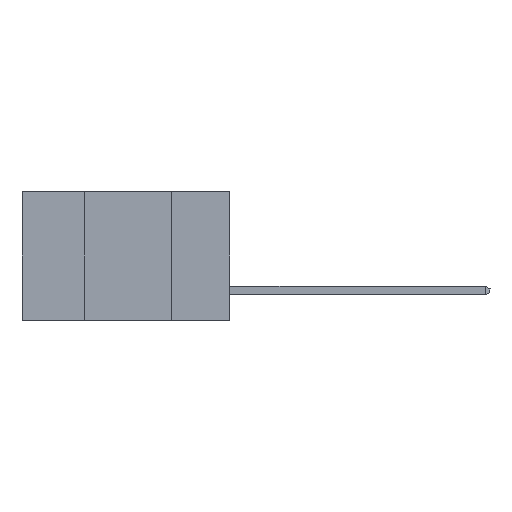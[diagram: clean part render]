
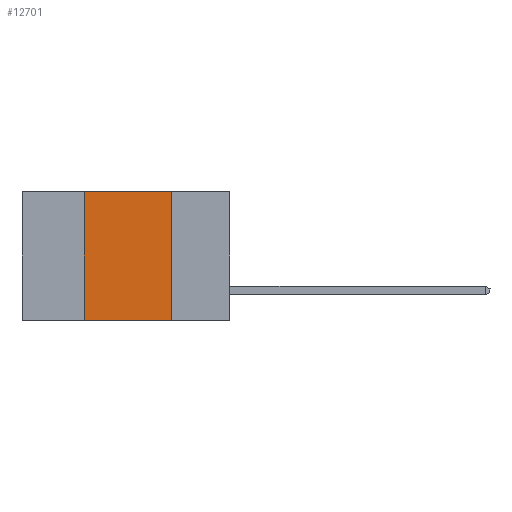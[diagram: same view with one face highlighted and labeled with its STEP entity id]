
A CAD part, left-side view. The second image highlights one B-rep face of the part: STEP entity #12701.
In plain terms, the highlighted planar face has unit normal (-1, 0, 0).
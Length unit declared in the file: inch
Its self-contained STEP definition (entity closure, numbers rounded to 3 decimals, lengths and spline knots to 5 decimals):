
#995 = DIRECTION ( 'NONE',  ( 0., 0., -1. ) ) ;
#1288 = CARTESIAN_POINT ( 'NONE',  ( 0., 0.42, 0. ) ) ;
#1943 = LINE ( 'NONE', #11636, #4097 ) ;
#1996 = DIRECTION ( 'NONE',  ( 0., 0., -1. ) ) ;
#2023 = CARTESIAN_POINT ( 'NONE',  ( 0., 0.42, -0.37 ) ) ;
#2169 = CARTESIAN_POINT ( 'NONE',  ( 0., 0.6, 0. ) ) ;
#2210 = LINE ( 'NONE', #11900, #9427 ) ;
#2412 = EDGE_CURVE ( 'NONE', #7372, #12033, #1943, .T. ) ;
#2417 = VECTOR ( 'NONE', #4695, 39.37008 ) ;
#2728 = ORIENTED_EDGE ( 'NONE', *, *, #10394, .F. ) ;
#3647 = EDGE_LOOP ( 'NONE', ( #7313, #10291, #2728, #4314 ) ) ;
#3679 = CARTESIAN_POINT ( 'NONE',  ( 0., 0.6, 0. ) ) ;
#3912 = CARTESIAN_POINT ( 'NONE',  ( 0., 0.17, -0.37 ) ) ;
#4097 = VECTOR ( 'NONE', #5203, 39.37008 ) ;
#4314 = ORIENTED_EDGE ( 'NONE', *, *, #2412, .T. ) ;
#4695 = DIRECTION ( 'NONE',  ( 0., -1., 0. ) ) ;
#5203 = DIRECTION ( 'NONE',  ( 0., -1., 0. ) ) ;
#6564 = LINE ( 'NONE', #7814, #9558 ) ;
#6735 = EDGE_CURVE ( 'NONE', #7533, #10564, #15694, .T. ) ;
#6776 = FACE_OUTER_BOUND ( 'NONE', #3647, .T. ) ;
#7313 = ORIENTED_EDGE ( 'NONE', *, *, #13667, .F. ) ;
#7372 = VERTEX_POINT ( 'NONE', #2023 ) ;
#7533 = VERTEX_POINT ( 'NONE', #1288 ) ;
#7744 = DIRECTION ( 'NONE',  ( 0., 0., 1. ) ) ;
#7814 = CARTESIAN_POINT ( 'NONE',  ( 0., 0.42, -0.37 ) ) ;
#9427 = VECTOR ( 'NONE', #995, 39.37008 ) ;
#9558 = VECTOR ( 'NONE', #7744, 39.37008 ) ;
#10291 = ORIENTED_EDGE ( 'NONE', *, *, #6735, .F. ) ;
#10394 = EDGE_CURVE ( 'NONE', #7372, #7533, #6564, .T. ) ;
#10564 = VERTEX_POINT ( 'NONE', #13186 ) ;
#10590 = DIRECTION ( 'NONE',  ( 1., 0., 0. ) ) ;
#11285 = AXIS2_PLACEMENT_3D ( 'NONE', #2169, #10590, #1996 ) ;
#11617 = PLANE ( 'NONE',  #11285 ) ;
#11636 = CARTESIAN_POINT ( 'NONE',  ( 0., 0.6, -0.37 ) ) ;
#11900 = CARTESIAN_POINT ( 'NONE',  ( 0., 0.17, -0.37 ) ) ;
#12033 = VERTEX_POINT ( 'NONE', #3912 ) ;
#12701 = ADVANCED_FACE ( 'NONE', ( #6776 ), #11617, .F. ) ;
#13186 = CARTESIAN_POINT ( 'NONE',  ( 0., 0.17, 0. ) ) ;
#13667 = EDGE_CURVE ( 'NONE', #10564, #12033, #2210, .T. ) ;
#15694 = LINE ( 'NONE', #3679, #2417 ) ;
